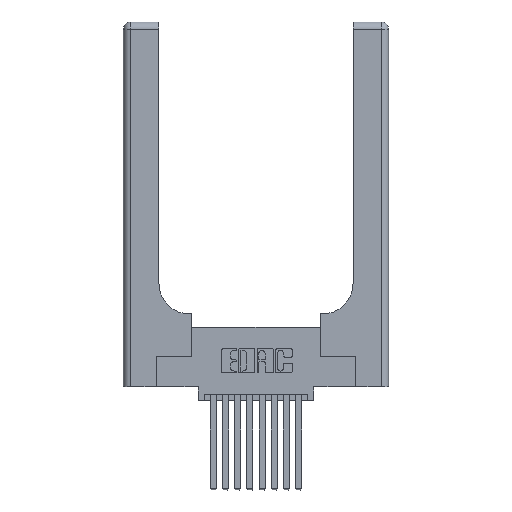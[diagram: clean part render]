
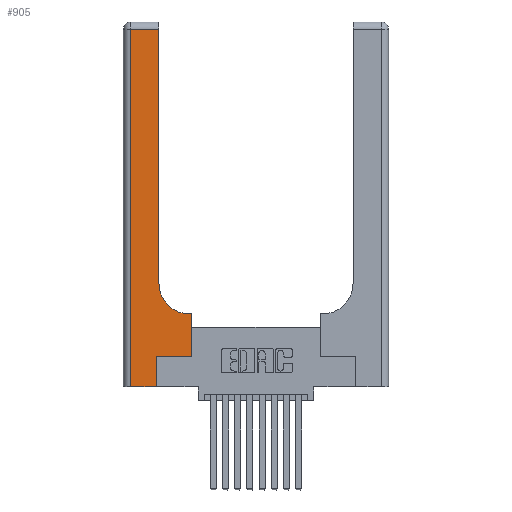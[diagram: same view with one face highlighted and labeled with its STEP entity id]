
A CAD part, top view. The second image highlights one B-rep face of the part: STEP entity #905.
In plain terms, the highlighted planar face has unit normal (0, 0, 1).
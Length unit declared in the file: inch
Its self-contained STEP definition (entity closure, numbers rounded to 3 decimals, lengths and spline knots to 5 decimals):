
#253 = VECTOR ( 'NONE', #10751, 39.37008 ) ;
#395 = ORIENTED_EDGE ( 'NONE', *, *, #11855, .T. ) ;
#551 = DIRECTION ( 'NONE',  ( 0., 1., 0. ) ) ;
#724 = CARTESIAN_POINT ( 'NONE',  ( 0.2915, 3., 0.37 ) ) ;
#905 = ADVANCED_FACE ( 'NONE', ( #15955 ), #13321, .F. ) ;
#1375 = CARTESIAN_POINT ( 'NONE',  ( 0.5585, 0.25, 0.37 ) ) ;
#1590 = VERTEX_POINT ( 'NONE', #6794 ) ;
#1743 = CARTESIAN_POINT ( 'NONE',  ( 0.269, 0.25, 0.37 ) ) ;
#1873 = LINE ( 'NONE', #12302, #11377 ) ;
#2040 = ORIENTED_EDGE ( 'NONE', *, *, #11488, .T. ) ;
#2163 = EDGE_CURVE ( 'NONE', #11718, #15038, #15739, .T. ) ;
#2604 = VECTOR ( 'NONE', #5287, 39.37008 ) ;
#2679 = DIRECTION ( 'NONE',  ( -1., 0., 0. ) ) ;
#2855 = VERTEX_POINT ( 'NONE', #10139 ) ;
#3063 = EDGE_LOOP ( 'NONE', ( #5966, #6347, #9598, #16008, #395, #4210, #7866, #14328, #2040 ) ) ;
#3144 = VECTOR ( 'NONE', #2679, 39.37008 ) ;
#3353 = CARTESIAN_POINT ( 'NONE',  ( 0.269, 0.25, 0.37 ) ) ;
#3683 = CARTESIAN_POINT ( 'NONE',  ( 0.06, 2.94, 0.37 ) ) ;
#3801 = EDGE_CURVE ( 'NONE', #7042, #7418, #10262, .T. ) ;
#3971 = DIRECTION ( 'NONE',  ( 0., -1., 0. ) ) ;
#3996 = VECTOR ( 'NONE', #11610, 39.37008 ) ;
#4210 = ORIENTED_EDGE ( 'NONE', *, *, #3801, .T. ) ;
#4413 = AXIS2_PLACEMENT_3D ( 'NONE', #13344, #13291, #13287 ) ;
#4889 = EDGE_CURVE ( 'NONE', #10743, #13848, #15109, .T. ) ;
#4954 = DIRECTION ( 'NONE',  ( 1., 0., 0. ) ) ;
#5023 = CARTESIAN_POINT ( 'NONE',  ( 0.06, 0., 0.37 ) ) ;
#5044 = CARTESIAN_POINT ( 'NONE',  ( 0.5415, 0.85, 0.37 ) ) ;
#5149 = CARTESIAN_POINT ( 'NONE',  ( 0.2915, 0.6, 0.37 ) ) ;
#5287 = DIRECTION ( 'NONE',  ( -1., 0., 0. ) ) ;
#5491 = CARTESIAN_POINT ( 'NONE',  ( 0.5585, 0.25, 0.37 ) ) ;
#5574 = CARTESIAN_POINT ( 'NONE',  ( 0.2915, 0.85, 0.37 ) ) ;
#5966 = ORIENTED_EDGE ( 'NONE', *, *, #2163, .T. ) ;
#6066 = VECTOR ( 'NONE', #551, 39.37008 ) ;
#6286 = DIRECTION ( 'NONE',  ( 1., 0., 0. ) ) ;
#6347 = ORIENTED_EDGE ( 'NONE', *, *, #6560, .T. ) ;
#6452 = LINE ( 'NONE', #5149, #3144 ) ;
#6560 = EDGE_CURVE ( 'NONE', #15038, #10743, #12461, .T. ) ;
#6794 = CARTESIAN_POINT ( 'NONE',  ( 0.5585, 0.6, 0.37 ) ) ;
#7042 = VERTEX_POINT ( 'NONE', #1743 ) ;
#7267 = DIRECTION ( 'NONE',  ( 0., 1., 0. ) ) ;
#7268 = LINE ( 'NONE', #5491, #3996 ) ;
#7418 = VERTEX_POINT ( 'NONE', #1375 ) ;
#7533 = AXIS2_PLACEMENT_3D ( 'NONE', #5044, #13590, #6286 ) ;
#7866 = ORIENTED_EDGE ( 'NONE', *, *, #12884, .T. ) ;
#8666 = VECTOR ( 'NONE', #3971, 39.37008 ) ;
#8846 = CARTESIAN_POINT ( 'NONE',  ( 0.2915, 2.94, 0.37 ) ) ;
#9598 = ORIENTED_EDGE ( 'NONE', *, *, #4889, .T. ) ;
#9613 = EDGE_CURVE ( 'NONE', #1590, #13279, #6452, .T. ) ;
#10139 = CARTESIAN_POINT ( 'NONE',  ( 0.269, 0., 0.37 ) ) ;
#10262 = LINE ( 'NONE', #3353, #253 ) ;
#10743 = VERTEX_POINT ( 'NONE', #3683 ) ;
#10750 = EDGE_CURVE ( 'NONE', #13848, #2855, #1873, .T. ) ;
#10751 = DIRECTION ( 'NONE',  ( 1., 0., 0. ) ) ;
#11000 = CIRCLE ( 'NONE', #7533, 0.25 ) ;
#11377 = VECTOR ( 'NONE', #4954, 39.37008 ) ;
#11413 = CARTESIAN_POINT ( 'NONE',  ( 0., 2.94, 0.37 ) ) ;
#11488 = EDGE_CURVE ( 'NONE', #13279, #11718, #11000, .T. ) ;
#11610 = DIRECTION ( 'NONE',  ( 0., 1., 0. ) ) ;
#11718 = VERTEX_POINT ( 'NONE', #5574 ) ;
#11855 = EDGE_CURVE ( 'NONE', #2855, #7042, #12500, .T. ) ;
#12283 = CARTESIAN_POINT ( 'NONE',  ( 0.5415, 0.6, 0.37 ) ) ;
#12302 = CARTESIAN_POINT ( 'NONE',  ( 0., 0., 0.37 ) ) ;
#12461 = LINE ( 'NONE', #11413, #2604 ) ;
#12500 = LINE ( 'NONE', #13378, #15285 ) ;
#12884 = EDGE_CURVE ( 'NONE', #7418, #1590, #7268, .T. ) ;
#13279 = VERTEX_POINT ( 'NONE', #12283 ) ;
#13287 = DIRECTION ( 'NONE',  ( -1., 0., 0. ) ) ;
#13291 = DIRECTION ( 'NONE',  ( 0., 0., -1. ) ) ;
#13321 = PLANE ( 'NONE',  #4413 ) ;
#13344 = CARTESIAN_POINT ( 'NONE',  ( 0., 3., 0.37 ) ) ;
#13378 = CARTESIAN_POINT ( 'NONE',  ( 0.269, 0., 0.37 ) ) ;
#13590 = DIRECTION ( 'NONE',  ( 0., 0., -1. ) ) ;
#13769 = CARTESIAN_POINT ( 'NONE',  ( 0.06, 3., 0.37 ) ) ;
#13848 = VERTEX_POINT ( 'NONE', #5023 ) ;
#14328 = ORIENTED_EDGE ( 'NONE', *, *, #9613, .T. ) ;
#15038 = VERTEX_POINT ( 'NONE', #8846 ) ;
#15109 = LINE ( 'NONE', #13769, #8666 ) ;
#15285 = VECTOR ( 'NONE', #7267, 39.37008 ) ;
#15739 = LINE ( 'NONE', #724, #6066 ) ;
#15955 = FACE_OUTER_BOUND ( 'NONE', #3063, .T. ) ;
#16008 = ORIENTED_EDGE ( 'NONE', *, *, #10750, .T. ) ;
